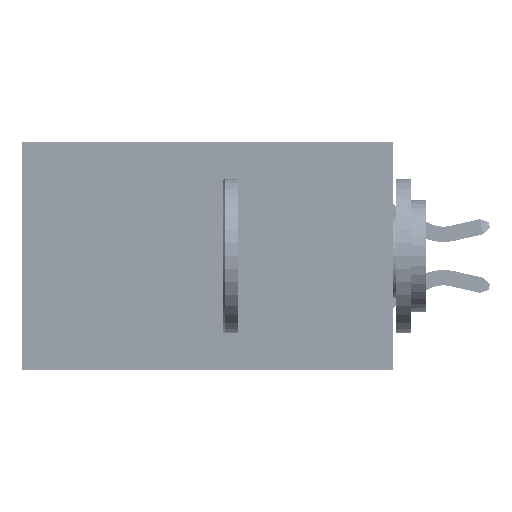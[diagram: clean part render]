
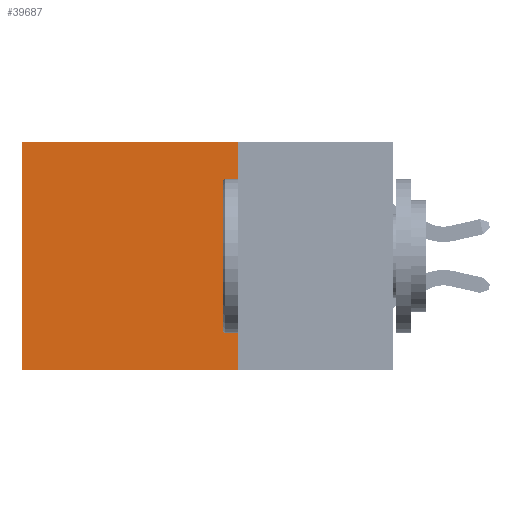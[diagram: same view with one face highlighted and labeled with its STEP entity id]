
A CAD part, left-side view. The second image highlights one B-rep face of the part: STEP entity #39687.
In plain terms, the highlighted planar face has unit normal (-1, 0, 0).
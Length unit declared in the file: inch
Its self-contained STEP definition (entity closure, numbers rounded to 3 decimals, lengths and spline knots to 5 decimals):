
#999 = EDGE_CURVE ( 'NONE', #47644, #17499, #46756, .T. ) ;
#1844 = EDGE_CURVE ( 'NONE', #15953, #4847, #6583, .T. ) ;
#2650 = VECTOR ( 'NONE', #38843, 39.37008 ) ;
#2823 = CARTESIAN_POINT ( 'NONE',  ( 0.2875, 0.6, -0.37 ) ) ;
#4262 = ORIENTED_EDGE ( 'NONE', *, *, #45380, .T. ) ;
#4847 = VERTEX_POINT ( 'NONE', #44818 ) ;
#6024 = DIRECTION ( 'NONE',  ( 0., 0., -1. ) ) ;
#6583 = LINE ( 'NONE', #30673, #13634 ) ;
#6919 = ORIENTED_EDGE ( 'NONE', *, *, #12355, .F. ) ;
#8359 = CARTESIAN_POINT ( 'NONE',  ( 0.2875, 0.25, 0. ) ) ;
#10000 = CARTESIAN_POINT ( 'NONE',  ( 0.2875, 0.25, 0. ) ) ;
#12355 = EDGE_CURVE ( 'NONE', #4847, #17499, #42756, .T. ) ;
#13634 = VECTOR ( 'NONE', #31467, 39.37008 ) ;
#14316 = DIRECTION ( 'NONE',  ( 0., 0., -1. ) ) ;
#15384 = ORIENTED_EDGE ( 'NONE', *, *, #999, .T. ) ;
#15953 = VERTEX_POINT ( 'NONE', #41688 ) ;
#17499 = VERTEX_POINT ( 'NONE', #2823 ) ;
#20048 = CARTESIAN_POINT ( 'NONE',  ( 0.2875, 0.25, -0.37 ) ) ;
#23789 = LINE ( 'NONE', #8359, #30255 ) ;
#28887 = PLANE ( 'NONE',  #29161 ) ;
#29161 = AXIS2_PLACEMENT_3D ( 'NONE', #10000, #43885, #6024 ) ;
#29594 = CARTESIAN_POINT ( 'NONE',  ( 0.2875, 0.6, 0. ) ) ;
#30255 = VECTOR ( 'NONE', #34196, 39.37008 ) ;
#30673 = CARTESIAN_POINT ( 'NONE',  ( 0.2875, 0.25, 0. ) ) ;
#31467 = DIRECTION ( 'NONE',  ( 0., 0., -1. ) ) ;
#34196 = DIRECTION ( 'NONE',  ( 0., 1., 0. ) ) ;
#35549 = VECTOR ( 'NONE', #14316, 39.37008 ) ;
#38081 = EDGE_LOOP ( 'NONE', ( #15384, #6919, #39515, #4262 ) ) ;
#38843 = DIRECTION ( 'NONE',  ( 0., 1., 0. ) ) ;
#39270 = FACE_OUTER_BOUND ( 'NONE', #38081, .T. ) ;
#39515 = ORIENTED_EDGE ( 'NONE', *, *, #1844, .F. ) ;
#39687 = ADVANCED_FACE ( 'NONE', ( #39270 ), #28887, .F. ) ;
#40958 = CARTESIAN_POINT ( 'NONE',  ( 0.2875, 0.6, 0. ) ) ;
#41688 = CARTESIAN_POINT ( 'NONE',  ( 0.2875, 0.25, 0. ) ) ;
#42756 = LINE ( 'NONE', #20048, #2650 ) ;
#43885 = DIRECTION ( 'NONE',  ( 1., 0., 0. ) ) ;
#44818 = CARTESIAN_POINT ( 'NONE',  ( 0.2875, 0.25, -0.37 ) ) ;
#45380 = EDGE_CURVE ( 'NONE', #15953, #47644, #23789, .T. ) ;
#46756 = LINE ( 'NONE', #29594, #35549 ) ;
#47644 = VERTEX_POINT ( 'NONE', #40958 ) ;
